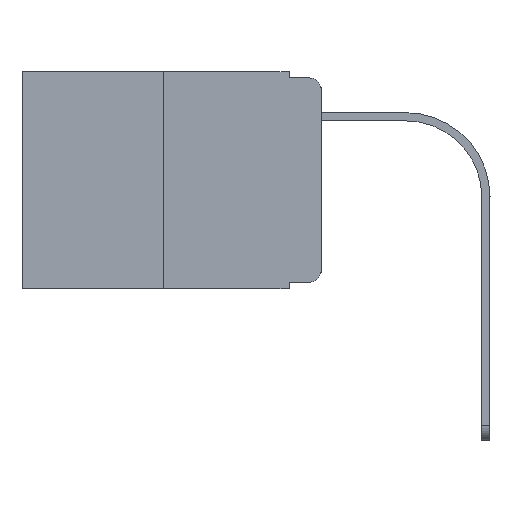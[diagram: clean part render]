
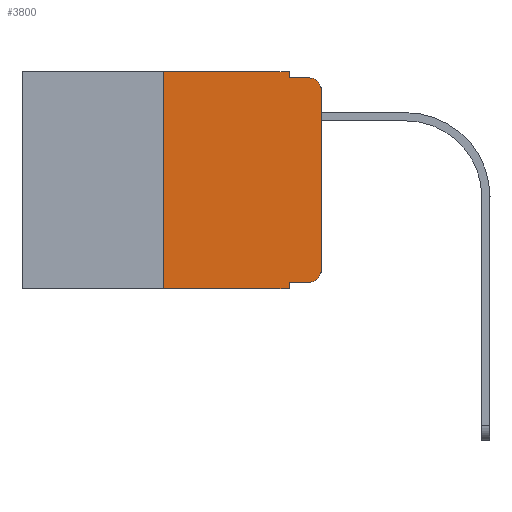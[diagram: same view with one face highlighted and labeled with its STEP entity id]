
A CAD part, left-side view. The second image highlights one B-rep face of the part: STEP entity #3800.
In plain terms, the highlighted planar face has unit normal (-1, 0, 0).
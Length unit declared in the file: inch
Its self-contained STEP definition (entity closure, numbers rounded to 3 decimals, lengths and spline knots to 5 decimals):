
#67 = VERTEX_POINT ( 'NONE', #6191 ) ;
#114 = AXIS2_PLACEMENT_3D ( 'NONE', #8343, #8114, #3124 ) ;
#216 = ORIENTED_EDGE ( 'NONE', *, *, #10414, .F. ) ;
#230 = CARTESIAN_POINT ( 'NONE',  ( 0., 0.051, -0.01 ) ) ;
#287 = CARTESIAN_POINT ( 'NONE',  ( 0., 0.02, -0.333 ) ) ;
#324 = LINE ( 'NONE', #7953, #3061 ) ;
#643 = ORIENTED_EDGE ( 'NONE', *, *, #2013, .F. ) ;
#664 = DIRECTION ( 'NONE',  ( -1., 0., 0. ) ) ;
#669 = CARTESIAN_POINT ( 'NONE',  ( 0., 0.051, 0. ) ) ;
#758 = VERTEX_POINT ( 'NONE', #5494 ) ;
#1215 = CARTESIAN_POINT ( 'NONE',  ( 0., 0.25, 0. ) ) ;
#1764 = LINE ( 'NONE', #6854, #10085 ) ;
#1874 = EDGE_CURVE ( 'NONE', #2572, #67, #8437, .T. ) ;
#1946 = ORIENTED_EDGE ( 'NONE', *, *, #9958, .T. ) ;
#2013 = EDGE_CURVE ( 'NONE', #4640, #7516, #2027, .T. ) ;
#2027 = LINE ( 'NONE', #5367, #2825 ) ;
#2092 = DIRECTION ( 'NONE',  ( 0., -1., 0. ) ) ;
#2311 = EDGE_CURVE ( 'NONE', #67, #758, #7986, .T. ) ;
#2572 = VERTEX_POINT ( 'NONE', #287 ) ;
#2583 = CARTESIAN_POINT ( 'NONE',  ( 0., 0.473, -0.343 ) ) ;
#2603 = CARTESIAN_POINT ( 'NONE',  ( 0., 0.051, 0. ) ) ;
#2617 = VECTOR ( 'NONE', #2748, 39.37008 ) ;
#2644 = ORIENTED_EDGE ( 'NONE', *, *, #9800, .F. ) ;
#2748 = DIRECTION ( 'NONE',  ( 0., -1., 0. ) ) ;
#2780 = CARTESIAN_POINT ( 'NONE',  ( 0., 0.25, -0.343 ) ) ;
#2825 = VECTOR ( 'NONE', #8723, 39.37008 ) ;
#2929 = VECTOR ( 'NONE', #6416, 39.37008 ) ;
#3061 = VECTOR ( 'NONE', #2092, 39.37008 ) ;
#3124 = DIRECTION ( 'NONE',  ( 0., 0., -1. ) ) ;
#3463 = VERTEX_POINT ( 'NONE', #3971 ) ;
#3470 = VERTEX_POINT ( 'NONE', #5805 ) ;
#3661 = LINE ( 'NONE', #1215, #8175 ) ;
#3670 = EDGE_CURVE ( 'NONE', #9086, #4640, #3661, .T. ) ;
#3800 = ADVANCED_FACE ( 'NONE', ( #3935 ), #4048, .F. ) ;
#3882 = DIRECTION ( 'NONE',  ( 0., 0., -1. ) ) ;
#3935 = FACE_OUTER_BOUND ( 'NONE', #6947, .T. ) ;
#3971 = CARTESIAN_POINT ( 'NONE',  ( 0., 0.051, -0.343 ) ) ;
#4048 = PLANE ( 'NONE',  #114 ) ;
#4141 = ORIENTED_EDGE ( 'NONE', *, *, #5906, .F. ) ;
#4556 = AXIS2_PLACEMENT_3D ( 'NONE', #6496, #664, #3882 ) ;
#4601 = AXIS2_PLACEMENT_3D ( 'NONE', #9686, #6302, #9742 ) ;
#4640 = VERTEX_POINT ( 'NONE', #9739 ) ;
#4667 = ORIENTED_EDGE ( 'NONE', *, *, #8503, .T. ) ;
#4944 = VERTEX_POINT ( 'NONE', #230 ) ;
#5019 = ORIENTED_EDGE ( 'NONE', *, *, #1874, .T. ) ;
#5063 = LINE ( 'NONE', #2603, #10325 ) ;
#5233 = VECTOR ( 'NONE', #9076, 39.37008 ) ;
#5367 = CARTESIAN_POINT ( 'NONE',  ( 0., 0.473, 0. ) ) ;
#5494 = CARTESIAN_POINT ( 'NONE',  ( 0., 0., -0.03 ) ) ;
#5547 = DIRECTION ( 'NONE',  ( 0., 0., 1. ) ) ;
#5805 = CARTESIAN_POINT ( 'NONE',  ( 0., 0.051, -0.333 ) ) ;
#5905 = DIRECTION ( 'NONE',  ( 0., 0., -1. ) ) ;
#5906 = EDGE_CURVE ( 'NONE', #7516, #4944, #5063, .T. ) ;
#5999 = LINE ( 'NONE', #2583, #2617 ) ;
#6191 = CARTESIAN_POINT ( 'NONE',  ( 0., 0., -0.313 ) ) ;
#6302 = DIRECTION ( 'NONE',  ( -1., 0., 0. ) ) ;
#6362 = VERTEX_POINT ( 'NONE', #9763 ) ;
#6416 = DIRECTION ( 'NONE',  ( 0., 0., 1. ) ) ;
#6496 = CARTESIAN_POINT ( 'NONE',  ( 0., 0.02, -0.313 ) ) ;
#6854 = CARTESIAN_POINT ( 'NONE',  ( 0., 0.051, -0.01 ) ) ;
#6947 = EDGE_LOOP ( 'NONE', ( #7710, #8994, #216, #4141, #643, #9485, #1946, #2644, #4667, #5019 ) ) ;
#7516 = VERTEX_POINT ( 'NONE', #9033 ) ;
#7710 = ORIENTED_EDGE ( 'NONE', *, *, #2311, .T. ) ;
#7953 = CARTESIAN_POINT ( 'NONE',  ( 0., 0.051, -0.333 ) ) ;
#7986 = LINE ( 'NONE', #8873, #2929 ) ;
#8114 = DIRECTION ( 'NONE',  ( 1., 0., 0. ) ) ;
#8175 = VECTOR ( 'NONE', #5547, 39.37008 ) ;
#8243 = EDGE_CURVE ( 'NONE', #758, #6362, #9347, .T. ) ;
#8247 = LINE ( 'NONE', #669, #5233 ) ;
#8341 = DIRECTION ( 'NONE',  ( 0., -1., 0. ) ) ;
#8343 = CARTESIAN_POINT ( 'NONE',  ( 0., 0.473, 0. ) ) ;
#8437 = CIRCLE ( 'NONE', #4556, 0.02 ) ;
#8503 = EDGE_CURVE ( 'NONE', #3470, #2572, #324, .T. ) ;
#8723 = DIRECTION ( 'NONE',  ( 0., -1., 0. ) ) ;
#8873 = CARTESIAN_POINT ( 'NONE',  ( 0., 0., 0. ) ) ;
#8994 = ORIENTED_EDGE ( 'NONE', *, *, #8243, .T. ) ;
#9033 = CARTESIAN_POINT ( 'NONE',  ( 0., 0.051, 0. ) ) ;
#9076 = DIRECTION ( 'NONE',  ( 0., 0., -1. ) ) ;
#9086 = VERTEX_POINT ( 'NONE', #2780 ) ;
#9347 = CIRCLE ( 'NONE', #4601, 0.02 ) ;
#9485 = ORIENTED_EDGE ( 'NONE', *, *, #3670, .F. ) ;
#9686 = CARTESIAN_POINT ( 'NONE',  ( 0., 0.02, -0.03 ) ) ;
#9739 = CARTESIAN_POINT ( 'NONE',  ( 0., 0.25, 0. ) ) ;
#9742 = DIRECTION ( 'NONE',  ( 0., 0., -1. ) ) ;
#9763 = CARTESIAN_POINT ( 'NONE',  ( 0., 0.02, -0.01 ) ) ;
#9800 = EDGE_CURVE ( 'NONE', #3470, #3463, #8247, .T. ) ;
#9958 = EDGE_CURVE ( 'NONE', #9086, #3463, #5999, .T. ) ;
#10085 = VECTOR ( 'NONE', #8341, 39.37008 ) ;
#10325 = VECTOR ( 'NONE', #5905, 39.37008 ) ;
#10414 = EDGE_CURVE ( 'NONE', #4944, #6362, #1764, .T. ) ;
